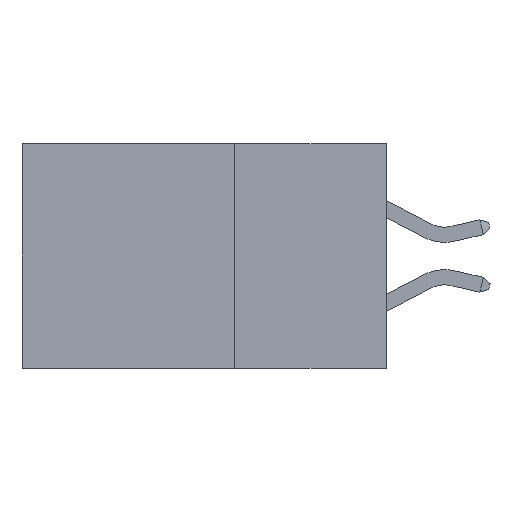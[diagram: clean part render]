
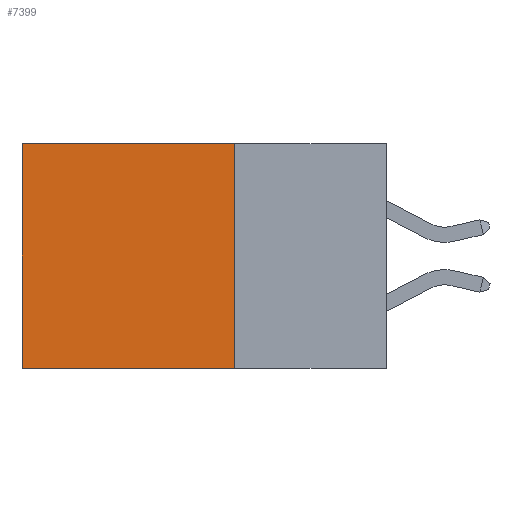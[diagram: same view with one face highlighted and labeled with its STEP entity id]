
A CAD part, left-side view. The second image highlights one B-rep face of the part: STEP entity #7399.
In plain terms, the highlighted planar face has unit normal (-1, 0, 0).
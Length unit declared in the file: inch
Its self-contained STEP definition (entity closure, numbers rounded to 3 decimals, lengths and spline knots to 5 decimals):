
#98 = PLANE ( 'NONE',  #6726 ) ;
#397 = VECTOR ( 'NONE', #8040, 39.37008 ) ;
#524 = EDGE_CURVE ( 'NONE', #8001, #3720, #1532, .T. ) ;
#860 = CARTESIAN_POINT ( 'NONE',  ( 0.298, 0.25, -0.37 ) ) ;
#1532 = LINE ( 'NONE', #3425, #9668 ) ;
#1627 = VERTEX_POINT ( 'NONE', #7306 ) ;
#1644 = CARTESIAN_POINT ( 'NONE',  ( 0.298, 0.25, 0. ) ) ;
#2010 = ORIENTED_EDGE ( 'NONE', *, *, #6082, .F. ) ;
#2119 = CARTESIAN_POINT ( 'NONE',  ( 0.298, 0.6, -0.37 ) ) ;
#2893 = FACE_OUTER_BOUND ( 'NONE', #3618, .T. ) ;
#2922 = CARTESIAN_POINT ( 'NONE',  ( 0.298, 0.25, 0. ) ) ;
#3069 = ORIENTED_EDGE ( 'NONE', *, *, #524, .T. ) ;
#3425 = CARTESIAN_POINT ( 'NONE',  ( 0.298, 0.6, 0. ) ) ;
#3580 = LINE ( 'NONE', #2922, #7287 ) ;
#3618 = EDGE_LOOP ( 'NONE', ( #3069, #2010, #6737, #8089 ) ) ;
#3720 = VERTEX_POINT ( 'NONE', #2119 ) ;
#3850 = EDGE_CURVE ( 'NONE', #1627, #8001, #3580, .T. ) ;
#4149 = CARTESIAN_POINT ( 'NONE',  ( 0.298, 0.25, -0.37 ) ) ;
#4275 = VERTEX_POINT ( 'NONE', #4149 ) ;
#5166 = CARTESIAN_POINT ( 'NONE',  ( 0.298, 0.25, 0. ) ) ;
#5641 = LINE ( 'NONE', #860, #397 ) ;
#6082 = EDGE_CURVE ( 'NONE', #4275, #3720, #5641, .T. ) ;
#6652 = CARTESIAN_POINT ( 'NONE',  ( 0.298, 0.6, 0. ) ) ;
#6726 = AXIS2_PLACEMENT_3D ( 'NONE', #1644, #7135, #7955 ) ;
#6737 = ORIENTED_EDGE ( 'NONE', *, *, #9349, .F. ) ;
#6912 = VECTOR ( 'NONE', #6972, 39.37008 ) ;
#6972 = DIRECTION ( 'NONE',  ( 0., 0., -1. ) ) ;
#7135 = DIRECTION ( 'NONE',  ( 1., 0., 0. ) ) ;
#7287 = VECTOR ( 'NONE', #9382, 39.37008 ) ;
#7306 = CARTESIAN_POINT ( 'NONE',  ( 0.298, 0.25, 0. ) ) ;
#7399 = ADVANCED_FACE ( 'NONE', ( #2893 ), #98, .F. ) ;
#7955 = DIRECTION ( 'NONE',  ( 0., 0., -1. ) ) ;
#8001 = VERTEX_POINT ( 'NONE', #6652 ) ;
#8040 = DIRECTION ( 'NONE',  ( 0., 1., 0. ) ) ;
#8089 = ORIENTED_EDGE ( 'NONE', *, *, #3850, .T. ) ;
#8784 = LINE ( 'NONE', #5166, #6912 ) ;
#9093 = DIRECTION ( 'NONE',  ( 0., 0., -1. ) ) ;
#9349 = EDGE_CURVE ( 'NONE', #1627, #4275, #8784, .T. ) ;
#9382 = DIRECTION ( 'NONE',  ( 0., 1., 0. ) ) ;
#9668 = VECTOR ( 'NONE', #9093, 39.37008 ) ;
